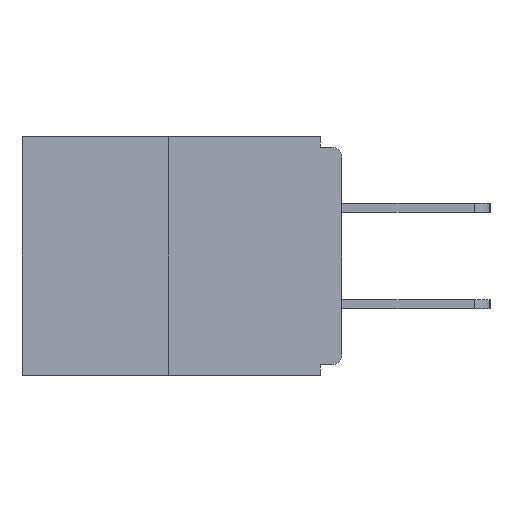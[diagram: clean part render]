
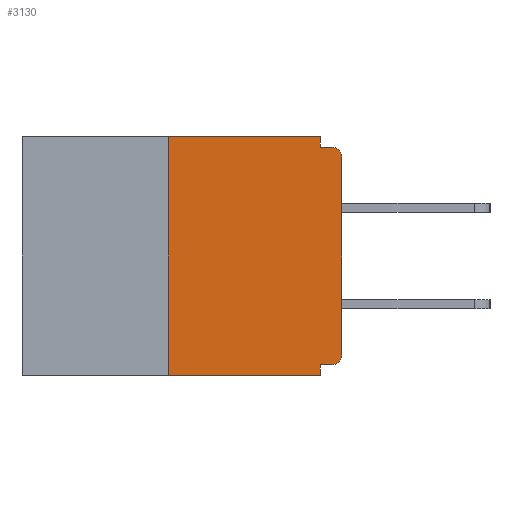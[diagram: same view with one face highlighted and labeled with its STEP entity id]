
A CAD part, left-side view. The second image highlights one B-rep face of the part: STEP entity #3130.
In plain terms, the highlighted planar face has unit normal (-1, 0, 0).
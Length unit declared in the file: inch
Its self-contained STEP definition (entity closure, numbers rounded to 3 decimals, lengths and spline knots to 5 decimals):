
#216 = CARTESIAN_POINT ( 'NONE',  ( 0., 0.015, -0.015 ) ) ;
#226 = AXIS2_PLACEMENT_3D ( 'NONE', #9034, #18846, #16611 ) ;
#350 = DIRECTION ( 'NONE',  ( -1., 0., 0. ) ) ;
#726 = VECTOR ( 'NONE', #19502, 39.37008 ) ;
#1091 = DIRECTION ( 'NONE',  ( -1., 0., 0. ) ) ;
#1840 = EDGE_CURVE ( 'NONE', #20614, #20010, #18318, .T. ) ;
#2572 = VERTEX_POINT ( 'NONE', #23422 ) ;
#2687 = DIRECTION ( 'NONE',  ( 0., 0., -1. ) ) ;
#3029 = DIRECTION ( 'NONE',  ( 0., 0., -1. ) ) ;
#3130 = ADVANCED_FACE ( 'NONE', ( #17635 ), #8795, .F. ) ;
#3135 = EDGE_CURVE ( 'NONE', #6933, #20614, #6052, .T. ) ;
#3244 = EDGE_CURVE ( 'NONE', #6100, #20010, #22209, .T. ) ;
#3313 = CARTESIAN_POINT ( 'NONE',  ( 0., 0.031, -0.343 ) ) ;
#3361 = DIRECTION ( 'NONE',  ( 0., -1., 0. ) ) ;
#3641 = CARTESIAN_POINT ( 'NONE',  ( 0., 0.25, 0. ) ) ;
#3944 = VECTOR ( 'NONE', #3361, 39.37008 ) ;
#4245 = VERTEX_POINT ( 'NONE', #7723 ) ;
#4699 = EDGE_LOOP ( 'NONE', ( #22697, #18723, #13880, #15616, #20605, #11264, #16727, #7317, #8806, #13619 ) ) ;
#5380 = CARTESIAN_POINT ( 'NONE',  ( 0., 0.46, -0.343 ) ) ;
#5815 = CARTESIAN_POINT ( 'NONE',  ( 0., 0., 0. ) ) ;
#6052 = LINE ( 'NONE', #8869, #12448 ) ;
#6100 = VERTEX_POINT ( 'NONE', #23368 ) ;
#6925 = EDGE_CURVE ( 'NONE', #10644, #2572, #23702, .T. ) ;
#6933 = VERTEX_POINT ( 'NONE', #14616 ) ;
#7317 = ORIENTED_EDGE ( 'NONE', *, *, #16243, .T. ) ;
#7421 = AXIS2_PLACEMENT_3D ( 'NONE', #7970, #350, #21611 ) ;
#7647 = DIRECTION ( 'NONE',  ( 0., 0., -1. ) ) ;
#7723 = CARTESIAN_POINT ( 'NONE',  ( 0., 0.031, -0.015 ) ) ;
#7970 = CARTESIAN_POINT ( 'NONE',  ( 0., 0.015, -0.03 ) ) ;
#8795 = PLANE ( 'NONE',  #226 ) ;
#8806 = ORIENTED_EDGE ( 'NONE', *, *, #22454, .F. ) ;
#8838 = DIRECTION ( 'NONE',  ( 0., 0., 1. ) ) ;
#8869 = CARTESIAN_POINT ( 'NONE',  ( 0., 0., -0.328 ) ) ;
#9034 = CARTESIAN_POINT ( 'NONE',  ( 0., 0.46, 0. ) ) ;
#9198 = LINE ( 'NONE', #13562, #726 ) ;
#9509 = VERTEX_POINT ( 'NONE', #216 ) ;
#10345 = AXIS2_PLACEMENT_3D ( 'NONE', #16772, #1091, #3029 ) ;
#10542 = CARTESIAN_POINT ( 'NONE',  ( 0., 0.46, 0. ) ) ;
#10644 = VERTEX_POINT ( 'NONE', #3641 ) ;
#11045 = CARTESIAN_POINT ( 'NONE',  ( 0., 0., -0.03 ) ) ;
#11215 = VECTOR ( 'NONE', #18547, 39.37008 ) ;
#11264 = ORIENTED_EDGE ( 'NONE', *, *, #14766, .T. ) ;
#11456 = CARTESIAN_POINT ( 'NONE',  ( 0., 0.031, -0.328 ) ) ;
#11485 = CIRCLE ( 'NONE', #10345, 0.015 ) ;
#11754 = DIRECTION ( 'NONE',  ( 0., 0., 1. ) ) ;
#12448 = VECTOR ( 'NONE', #22738, 39.37008 ) ;
#12910 = CIRCLE ( 'NONE', #7421, 0.015 ) ;
#13562 = CARTESIAN_POINT ( 'NONE',  ( 0., 0., -0.015 ) ) ;
#13619 = ORIENTED_EDGE ( 'NONE', *, *, #18380, .F. ) ;
#13880 = ORIENTED_EDGE ( 'NONE', *, *, #3244, .T. ) ;
#14301 = CARTESIAN_POINT ( 'NONE',  ( 0., 0.031, 0. ) ) ;
#14348 = VECTOR ( 'NONE', #7647, 39.37008 ) ;
#14616 = CARTESIAN_POINT ( 'NONE',  ( 0., 0.015, -0.328 ) ) ;
#14766 = EDGE_CURVE ( 'NONE', #6933, #23087, #11485, .T. ) ;
#15616 = ORIENTED_EDGE ( 'NONE', *, *, #1840, .F. ) ;
#16243 = EDGE_CURVE ( 'NONE', #18593, #9509, #12910, .T. ) ;
#16611 = DIRECTION ( 'NONE',  ( 0., 0., -1. ) ) ;
#16727 = ORIENTED_EDGE ( 'NONE', *, *, #21377, .T. ) ;
#16772 = CARTESIAN_POINT ( 'NONE',  ( 0., 0.015, -0.313 ) ) ;
#17214 = VECTOR ( 'NONE', #8838, 39.37008 ) ;
#17635 = FACE_OUTER_BOUND ( 'NONE', #4699, .T. ) ;
#18318 = LINE ( 'NONE', #21451, #14348 ) ;
#18380 = EDGE_CURVE ( 'NONE', #2572, #4245, #18865, .T. ) ;
#18547 = DIRECTION ( 'NONE',  ( 0., -1., 0. ) ) ;
#18593 = VERTEX_POINT ( 'NONE', #11045 ) ;
#18723 = ORIENTED_EDGE ( 'NONE', *, *, #20399, .F. ) ;
#18846 = DIRECTION ( 'NONE',  ( 1., 0., 0. ) ) ;
#18865 = LINE ( 'NONE', #14301, #23418 ) ;
#19046 = VECTOR ( 'NONE', #11754, 39.37008 ) ;
#19202 = CARTESIAN_POINT ( 'NONE',  ( 0., 0., -0.313 ) ) ;
#19502 = DIRECTION ( 'NONE',  ( 0., -1., 0. ) ) ;
#20010 = VERTEX_POINT ( 'NONE', #3313 ) ;
#20399 = EDGE_CURVE ( 'NONE', #6100, #10644, #22391, .T. ) ;
#20605 = ORIENTED_EDGE ( 'NONE', *, *, #3135, .F. ) ;
#20614 = VERTEX_POINT ( 'NONE', #11456 ) ;
#21377 = EDGE_CURVE ( 'NONE', #23087, #18593, #24196, .T. ) ;
#21451 = CARTESIAN_POINT ( 'NONE',  ( 0., 0.031, -0.343 ) ) ;
#21611 = DIRECTION ( 'NONE',  ( 0., 0., -1. ) ) ;
#22209 = LINE ( 'NONE', #5380, #3944 ) ;
#22391 = LINE ( 'NONE', #24235, #17214 ) ;
#22454 = EDGE_CURVE ( 'NONE', #4245, #9509, #9198, .T. ) ;
#22697 = ORIENTED_EDGE ( 'NONE', *, *, #6925, .F. ) ;
#22738 = DIRECTION ( 'NONE',  ( 0., 1., 0. ) ) ;
#23087 = VERTEX_POINT ( 'NONE', #19202 ) ;
#23368 = CARTESIAN_POINT ( 'NONE',  ( 0., 0.25, -0.343 ) ) ;
#23418 = VECTOR ( 'NONE', #2687, 39.37008 ) ;
#23422 = CARTESIAN_POINT ( 'NONE',  ( 0., 0.031, 0. ) ) ;
#23702 = LINE ( 'NONE', #10542, #11215 ) ;
#24196 = LINE ( 'NONE', #5815, #19046 ) ;
#24235 = CARTESIAN_POINT ( 'NONE',  ( 0., 0.25, 0. ) ) ;
